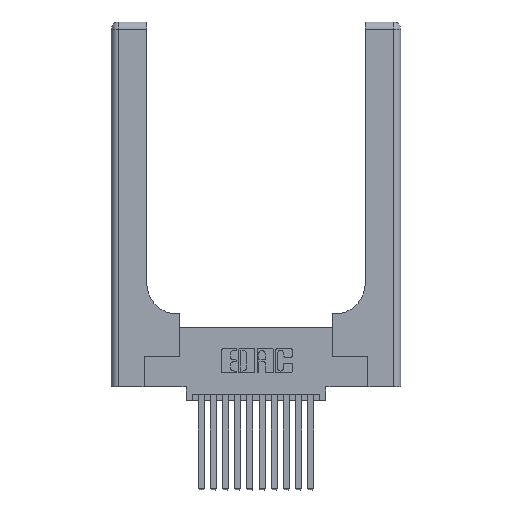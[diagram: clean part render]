
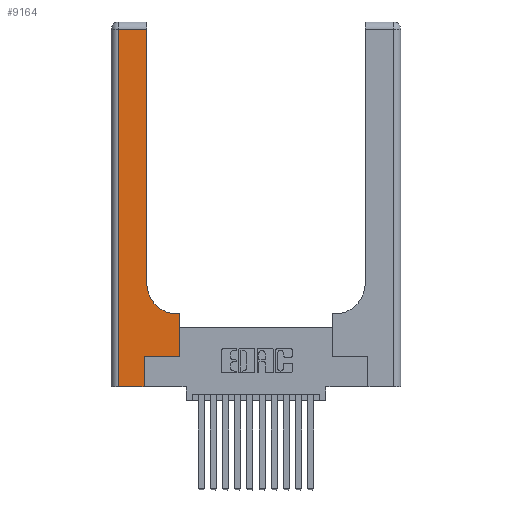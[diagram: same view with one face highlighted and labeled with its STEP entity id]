
A CAD part, top view. The second image highlights one B-rep face of the part: STEP entity #9164.
In plain terms, the highlighted planar face has unit normal (0, 0, 1).
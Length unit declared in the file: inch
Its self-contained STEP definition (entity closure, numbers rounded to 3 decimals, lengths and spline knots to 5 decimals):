
#496 = CARTESIAN_POINT ( 'NONE',  ( 0.5585, 0.25, 0.37 ) ) ;
#997 = VECTOR ( 'NONE', #10076, 39.37008 ) ;
#1027 = EDGE_CURVE ( 'NONE', #7444, #8157, #12151, .T. ) ;
#1502 = CARTESIAN_POINT ( 'NONE',  ( 0.06, 2.94, 0.37 ) ) ;
#1652 = DIRECTION ( 'NONE',  ( -1., 0., 0. ) ) ;
#1726 = VECTOR ( 'NONE', #8488, 39.37008 ) ;
#1851 = DIRECTION ( 'NONE',  ( 0., 1., 0. ) ) ;
#2060 = DIRECTION ( 'NONE',  ( 0., -1., 0. ) ) ;
#2958 = DIRECTION ( 'NONE',  ( 1., 0., 0. ) ) ;
#3455 = VERTEX_POINT ( 'NONE', #15277 ) ;
#3536 = EDGE_CURVE ( 'NONE', #8447, #7444, #4569, .T. ) ;
#3658 = CARTESIAN_POINT ( 'NONE',  ( 0., 3., 0.37 ) ) ;
#4035 = ORIENTED_EDGE ( 'NONE', *, *, #16020, .T. ) ;
#4220 = CARTESIAN_POINT ( 'NONE',  ( 0.2915, 0.85, 0.37 ) ) ;
#4461 = ORIENTED_EDGE ( 'NONE', *, *, #4578, .T. ) ;
#4569 = LINE ( 'NONE', #16729, #997 ) ;
#4578 = EDGE_CURVE ( 'NONE', #14731, #3455, #14825, .T. ) ;
#4658 = LINE ( 'NONE', #8753, #11343 ) ;
#4962 = EDGE_LOOP ( 'NONE', ( #9895, #16991, #6794, #13929, #4035, #4461, #11578, #15610, #5307 ) ) ;
#5011 = DIRECTION ( 'NONE',  ( -1., 0., 0. ) ) ;
#5132 = VECTOR ( 'NONE', #1851, 39.37008 ) ;
#5273 = EDGE_CURVE ( 'NONE', #7143, #17104, #8296, .T. ) ;
#5307 = ORIENTED_EDGE ( 'NONE', *, *, #1027, .T. ) ;
#5651 = CARTESIAN_POINT ( 'NONE',  ( 0., 2.94, 0.37 ) ) ;
#6353 = AXIS2_PLACEMENT_3D ( 'NONE', #3658, #13043, #5011 ) ;
#6735 = VECTOR ( 'NONE', #12796, 39.37008 ) ;
#6794 = ORIENTED_EDGE ( 'NONE', *, *, #9628, .T. ) ;
#7143 = VERTEX_POINT ( 'NONE', #12580 ) ;
#7440 = CARTESIAN_POINT ( 'NONE',  ( 0.2915, 3., 0.37 ) ) ;
#7444 = VERTEX_POINT ( 'NONE', #8085 ) ;
#7580 = LINE ( 'NONE', #7440, #6735 ) ;
#7654 = VECTOR ( 'NONE', #10237, 39.37008 ) ;
#7685 = DIRECTION ( 'NONE',  ( 1., 0., 0. ) ) ;
#7702 = VECTOR ( 'NONE', #2958, 39.37008 ) ;
#8085 = CARTESIAN_POINT ( 'NONE',  ( 0.5415, 0.6, 0.37 ) ) ;
#8157 = VERTEX_POINT ( 'NONE', #4220 ) ;
#8296 = LINE ( 'NONE', #5651, #11402 ) ;
#8412 = CARTESIAN_POINT ( 'NONE',  ( 0.269, 0.25, 0.37 ) ) ;
#8417 = DIRECTION ( 'NONE',  ( 0., 0., -1. ) ) ;
#8440 = CARTESIAN_POINT ( 'NONE',  ( 0.5415, 0.85, 0.37 ) ) ;
#8447 = VERTEX_POINT ( 'NONE', #15307 ) ;
#8488 = DIRECTION ( 'NONE',  ( 0., 1., 0. ) ) ;
#8724 = CARTESIAN_POINT ( 'NONE',  ( 0.06, 0., 0.37 ) ) ;
#8753 = CARTESIAN_POINT ( 'NONE',  ( 0.06, 3., 0.37 ) ) ;
#9164 = ADVANCED_FACE ( 'NONE', ( #17132 ), #11676, .F. ) ;
#9166 = VERTEX_POINT ( 'NONE', #10337 ) ;
#9581 = CARTESIAN_POINT ( 'NONE',  ( 0.269, 0.25, 0.37 ) ) ;
#9628 = EDGE_CURVE ( 'NONE', #17104, #14188, #4658, .T. ) ;
#9895 = ORIENTED_EDGE ( 'NONE', *, *, #10824, .T. ) ;
#10076 = DIRECTION ( 'NONE',  ( -1., 0., 0. ) ) ;
#10237 = DIRECTION ( 'NONE',  ( 1., 0., 0. ) ) ;
#10337 = CARTESIAN_POINT ( 'NONE',  ( 0.269, 0., 0.37 ) ) ;
#10824 = EDGE_CURVE ( 'NONE', #8157, #7143, #7580, .T. ) ;
#11343 = VECTOR ( 'NONE', #2060, 39.37008 ) ;
#11402 = VECTOR ( 'NONE', #1652, 39.37008 ) ;
#11578 = ORIENTED_EDGE ( 'NONE', *, *, #14108, .T. ) ;
#11586 = LINE ( 'NONE', #16825, #7654 ) ;
#11676 = PLANE ( 'NONE',  #6353 ) ;
#11994 = LINE ( 'NONE', #16480, #1726 ) ;
#12151 = CIRCLE ( 'NONE', #15689, 0.25 ) ;
#12580 = CARTESIAN_POINT ( 'NONE',  ( 0.2915, 2.94, 0.37 ) ) ;
#12796 = DIRECTION ( 'NONE',  ( 0., 1., 0. ) ) ;
#13043 = DIRECTION ( 'NONE',  ( 0., 0., -1. ) ) ;
#13929 = ORIENTED_EDGE ( 'NONE', *, *, #15634, .T. ) ;
#14108 = EDGE_CURVE ( 'NONE', #3455, #8447, #15830, .T. ) ;
#14188 = VERTEX_POINT ( 'NONE', #8724 ) ;
#14731 = VERTEX_POINT ( 'NONE', #8412 ) ;
#14825 = LINE ( 'NONE', #9581, #7702 ) ;
#15277 = CARTESIAN_POINT ( 'NONE',  ( 0.5585, 0.25, 0.37 ) ) ;
#15307 = CARTESIAN_POINT ( 'NONE',  ( 0.5585, 0.6, 0.37 ) ) ;
#15610 = ORIENTED_EDGE ( 'NONE', *, *, #3536, .T. ) ;
#15634 = EDGE_CURVE ( 'NONE', #14188, #9166, #11586, .T. ) ;
#15689 = AXIS2_PLACEMENT_3D ( 'NONE', #8440, #8417, #7685 ) ;
#15830 = LINE ( 'NONE', #496, #5132 ) ;
#16020 = EDGE_CURVE ( 'NONE', #9166, #14731, #11994, .T. ) ;
#16480 = CARTESIAN_POINT ( 'NONE',  ( 0.269, 0., 0.37 ) ) ;
#16729 = CARTESIAN_POINT ( 'NONE',  ( 0.2915, 0.6, 0.37 ) ) ;
#16825 = CARTESIAN_POINT ( 'NONE',  ( 0., 0., 0.37 ) ) ;
#16991 = ORIENTED_EDGE ( 'NONE', *, *, #5273, .T. ) ;
#17104 = VERTEX_POINT ( 'NONE', #1502 ) ;
#17132 = FACE_OUTER_BOUND ( 'NONE', #4962, .T. ) ;
